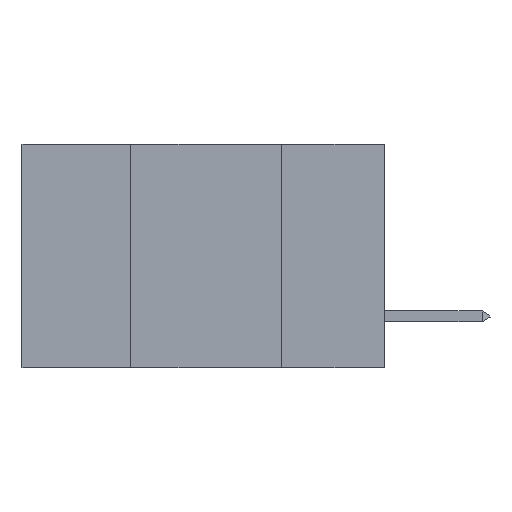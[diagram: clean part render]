
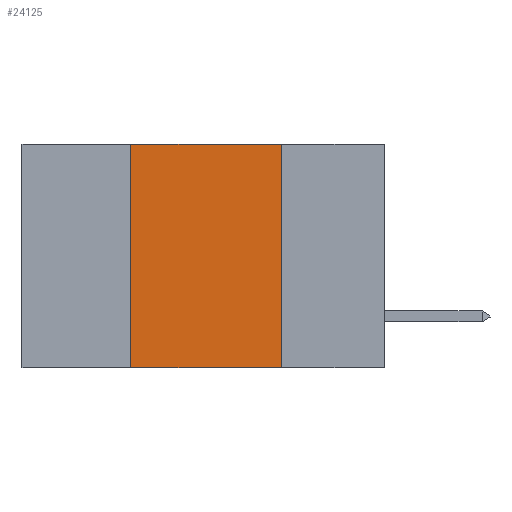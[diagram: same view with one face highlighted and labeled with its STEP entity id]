
A CAD part, left-side view. The second image highlights one B-rep face of the part: STEP entity #24125.
In plain terms, the highlighted planar face has unit normal (-1, 0, 0).
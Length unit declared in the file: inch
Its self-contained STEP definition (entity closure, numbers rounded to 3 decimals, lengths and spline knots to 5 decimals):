
#2251 = DIRECTION ( 'NONE',  ( 0., -1., 0. ) ) ;
#8340 = CARTESIAN_POINT ( 'NONE',  ( 0., 0.6, 0. ) ) ;
#10072 = EDGE_CURVE ( 'NONE', #18519, #29766, #25303, .T. ) ;
#12231 = ORIENTED_EDGE ( 'NONE', *, *, #16576, .F. ) ;
#13550 = EDGE_CURVE ( 'NONE', #29766, #14314, #21266, .T. ) ;
#14314 = VERTEX_POINT ( 'NONE', #19284 ) ;
#14547 = EDGE_LOOP ( 'NONE', ( #12231, #38178, #35954, #24936 ) ) ;
#16104 = VECTOR ( 'NONE', #37962, 39.37008 ) ;
#16576 = EDGE_CURVE ( 'NONE', #14314, #23797, #16631, .T. ) ;
#16631 = LINE ( 'NONE', #28418, #40539 ) ;
#17137 = CARTESIAN_POINT ( 'NONE',  ( 0., 0.42, 0. ) ) ;
#18519 = VERTEX_POINT ( 'NONE', #25670 ) ;
#19284 = CARTESIAN_POINT ( 'NONE',  ( 0., 0.17, 0. ) ) ;
#21266 = LINE ( 'NONE', #8340, #33825 ) ;
#23269 = AXIS2_PLACEMENT_3D ( 'NONE', #40994, #38377, #33652 ) ;
#23797 = VERTEX_POINT ( 'NONE', #29404 ) ;
#24125 = ADVANCED_FACE ( 'NONE', ( #34184 ), #24250, .F. ) ;
#24250 = PLANE ( 'NONE',  #23269 ) ;
#24936 = ORIENTED_EDGE ( 'NONE', *, *, #34717, .T. ) ;
#25303 = LINE ( 'NONE', #28561, #16104 ) ;
#25670 = CARTESIAN_POINT ( 'NONE',  ( 0., 0.42, -0.37 ) ) ;
#28418 = CARTESIAN_POINT ( 'NONE',  ( 0., 0.17, 0. ) ) ;
#28561 = CARTESIAN_POINT ( 'NONE',  ( 0., 0.42, 0. ) ) ;
#29404 = CARTESIAN_POINT ( 'NONE',  ( 0., 0.17, -0.37 ) ) ;
#29766 = VERTEX_POINT ( 'NONE', #17137 ) ;
#33652 = DIRECTION ( 'NONE',  ( 0., 0., -1. ) ) ;
#33825 = VECTOR ( 'NONE', #2251, 39.37008 ) ;
#34184 = FACE_OUTER_BOUND ( 'NONE', #14547, .T. ) ;
#34522 = CARTESIAN_POINT ( 'NONE',  ( 0., 0.6, -0.37 ) ) ;
#34717 = EDGE_CURVE ( 'NONE', #18519, #23797, #44265, .T. ) ;
#35954 = ORIENTED_EDGE ( 'NONE', *, *, #10072, .F. ) ;
#37962 = DIRECTION ( 'NONE',  ( 0., 0., 1. ) ) ;
#38178 = ORIENTED_EDGE ( 'NONE', *, *, #13550, .F. ) ;
#38377 = DIRECTION ( 'NONE',  ( 1., 0., 0. ) ) ;
#40539 = VECTOR ( 'NONE', #42451, 39.37008 ) ;
#40990 = DIRECTION ( 'NONE',  ( 0., -1., 0. ) ) ;
#40994 = CARTESIAN_POINT ( 'NONE',  ( 0., 0.6, 0. ) ) ;
#42451 = DIRECTION ( 'NONE',  ( 0., 0., -1. ) ) ;
#43744 = VECTOR ( 'NONE', #40990, 39.37008 ) ;
#44265 = LINE ( 'NONE', #34522, #43744 ) ;
